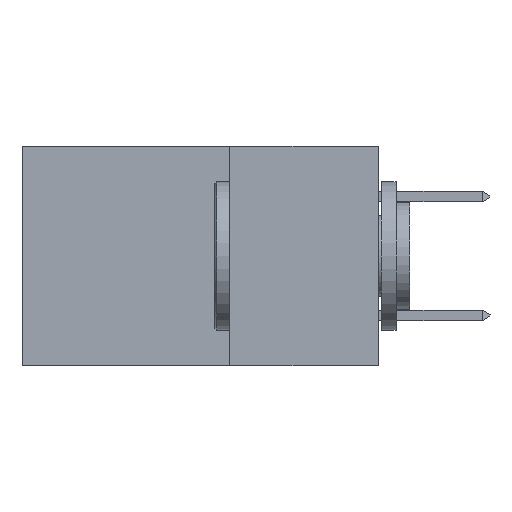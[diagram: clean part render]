
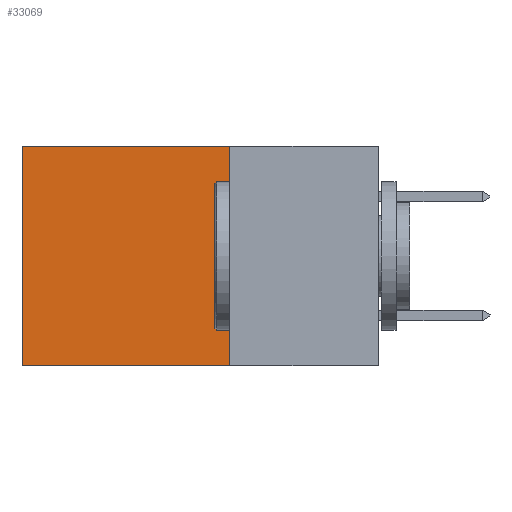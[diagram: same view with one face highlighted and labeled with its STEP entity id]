
A CAD part, left-side view. The second image highlights one B-rep face of the part: STEP entity #33069.
In plain terms, the highlighted planar face has unit normal (-1, 0, 0).
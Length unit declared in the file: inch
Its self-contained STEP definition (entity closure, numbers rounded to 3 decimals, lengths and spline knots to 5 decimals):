
#92 = LINE ( 'NONE', #14987, #11377 ) ;
#974 = CARTESIAN_POINT ( 'NONE',  ( 0.298, 0.25, 0. ) ) ;
#1572 = PLANE ( 'NONE',  #14128 ) ;
#1730 = CARTESIAN_POINT ( 'NONE',  ( 0.298, 0.25, -0.37 ) ) ;
#2279 = EDGE_LOOP ( 'NONE', ( #26141, #20092, #29492, #13806 ) ) ;
#5959 = CARTESIAN_POINT ( 'NONE',  ( 0.298, 0.25, 0. ) ) ;
#8032 = CARTESIAN_POINT ( 'NONE',  ( 0.298, 0.6, -0.37 ) ) ;
#8235 = EDGE_CURVE ( 'NONE', #10742, #23308, #14034, .T. ) ;
#10742 = VERTEX_POINT ( 'NONE', #5959 ) ;
#11377 = VECTOR ( 'NONE', #12744, 39.37008 ) ;
#11914 = DIRECTION ( 'NONE',  ( 1., 0., 0. ) ) ;
#12617 = DIRECTION ( 'NONE',  ( 0., 0., -1. ) ) ;
#12744 = DIRECTION ( 'NONE',  ( 0., 0., -1. ) ) ;
#13245 = EDGE_CURVE ( 'NONE', #10742, #19563, #20906, .T. ) ;
#13806 = ORIENTED_EDGE ( 'NONE', *, *, #13245, .T. ) ;
#13853 = VERTEX_POINT ( 'NONE', #8032 ) ;
#14034 = LINE ( 'NONE', #25567, #31757 ) ;
#14128 = AXIS2_PLACEMENT_3D ( 'NONE', #16943, #11914, #19338 ) ;
#14987 = CARTESIAN_POINT ( 'NONE',  ( 0.298, 0.6, 0. ) ) ;
#16003 = DIRECTION ( 'NONE',  ( 0., 1., 0. ) ) ;
#16842 = VECTOR ( 'NONE', #26528, 39.37008 ) ;
#16943 = CARTESIAN_POINT ( 'NONE',  ( 0.298, 0.25, 0. ) ) ;
#17293 = VECTOR ( 'NONE', #16003, 39.37008 ) ;
#19338 = DIRECTION ( 'NONE',  ( 0., 0., -1. ) ) ;
#19563 = VERTEX_POINT ( 'NONE', #19586 ) ;
#19586 = CARTESIAN_POINT ( 'NONE',  ( 0.298, 0.6, 0. ) ) ;
#20092 = ORIENTED_EDGE ( 'NONE', *, *, #24073, .F. ) ;
#20906 = LINE ( 'NONE', #974, #16842 ) ;
#21974 = EDGE_CURVE ( 'NONE', #19563, #13853, #92, .T. ) ;
#23308 = VERTEX_POINT ( 'NONE', #1730 ) ;
#24073 = EDGE_CURVE ( 'NONE', #23308, #13853, #31375, .T. ) ;
#25567 = CARTESIAN_POINT ( 'NONE',  ( 0.298, 0.25, 0. ) ) ;
#26141 = ORIENTED_EDGE ( 'NONE', *, *, #21974, .T. ) ;
#26528 = DIRECTION ( 'NONE',  ( 0., 1., 0. ) ) ;
#27598 = FACE_OUTER_BOUND ( 'NONE', #2279, .T. ) ;
#29294 = CARTESIAN_POINT ( 'NONE',  ( 0.298, 0.25, -0.37 ) ) ;
#29492 = ORIENTED_EDGE ( 'NONE', *, *, #8235, .F. ) ;
#31375 = LINE ( 'NONE', #29294, #17293 ) ;
#31757 = VECTOR ( 'NONE', #12617, 39.37008 ) ;
#33069 = ADVANCED_FACE ( 'NONE', ( #27598 ), #1572, .F. ) ;
